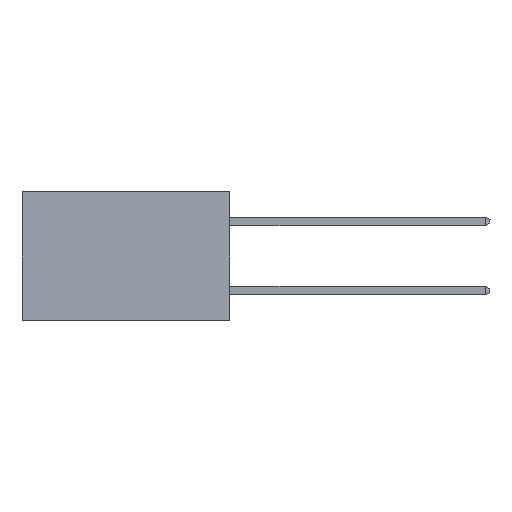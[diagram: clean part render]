
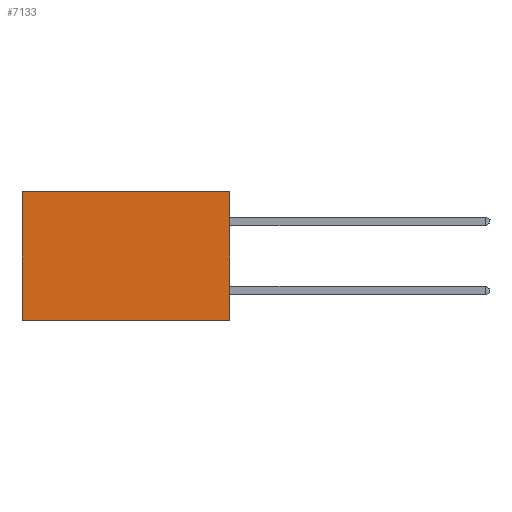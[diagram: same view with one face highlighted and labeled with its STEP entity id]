
A CAD part, left-side view. The second image highlights one B-rep face of the part: STEP entity #7133.
In plain terms, the highlighted planar face has unit normal (-1, 0, 0).
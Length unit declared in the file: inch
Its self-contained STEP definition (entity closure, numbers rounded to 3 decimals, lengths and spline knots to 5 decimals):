
#463 = ORIENTED_EDGE ( 'NONE', *, *, #21681, .F. ) ;
#1306 = FACE_OUTER_BOUND ( 'NONE', #14244, .T. ) ;
#1597 = VERTEX_POINT ( 'NONE', #17322 ) ;
#1683 = VECTOR ( 'NONE', #14192, 39.37008 ) ;
#1916 = PLANE ( 'NONE',  #7935 ) ;
#2069 = VERTEX_POINT ( 'NONE', #25078 ) ;
#2081 = LINE ( 'NONE', #17853, #12678 ) ;
#2197 = DIRECTION ( 'NONE',  ( 0., 0., -1. ) ) ;
#2674 = CARTESIAN_POINT ( 'NONE',  ( 0.2615, 0., -0.37 ) ) ;
#3080 = VECTOR ( 'NONE', #15954, 39.37008 ) ;
#6825 = VERTEX_POINT ( 'NONE', #20191 ) ;
#7133 = ADVANCED_FACE ( 'NONE', ( #1306 ), #1916, .F. ) ;
#7889 = ORIENTED_EDGE ( 'NONE', *, *, #12281, .T. ) ;
#7935 = AXIS2_PLACEMENT_3D ( 'NONE', #12000, #11866, #9193 ) ;
#8075 = CARTESIAN_POINT ( 'NONE',  ( 0.2615, 0., 0. ) ) ;
#9193 = DIRECTION ( 'NONE',  ( 0., 0., -1. ) ) ;
#11866 = DIRECTION ( 'NONE',  ( 1., 0., 0. ) ) ;
#12000 = CARTESIAN_POINT ( 'NONE',  ( 0.2615, 0., -0.37 ) ) ;
#12193 = LINE ( 'NONE', #8075, #3080 ) ;
#12235 = DIRECTION ( 'NONE',  ( 0., 0., -1. ) ) ;
#12281 = EDGE_CURVE ( 'NONE', #18769, #2069, #16241, .T. ) ;
#12386 = LINE ( 'NONE', #2674, #1683 ) ;
#12678 = VECTOR ( 'NONE', #2197, 39.37008 ) ;
#13939 = ORIENTED_EDGE ( 'NONE', *, *, #14836, .F. ) ;
#14192 = DIRECTION ( 'NONE',  ( 0., 1., 0. ) ) ;
#14244 = EDGE_LOOP ( 'NONE', ( #7889, #463, #13939, #14315 ) ) ;
#14315 = ORIENTED_EDGE ( 'NONE', *, *, #23627, .T. ) ;
#14667 = VECTOR ( 'NONE', #12235, 39.37008 ) ;
#14836 = EDGE_CURVE ( 'NONE', #1597, #6825, #2081, .T. ) ;
#15718 = CARTESIAN_POINT ( 'NONE',  ( 0.2615, 0.6, 0. ) ) ;
#15954 = DIRECTION ( 'NONE',  ( 0., 1., 0. ) ) ;
#16241 = LINE ( 'NONE', #16370, #14667 ) ;
#16370 = CARTESIAN_POINT ( 'NONE',  ( 0.2615, 0.6, -0.37 ) ) ;
#17322 = CARTESIAN_POINT ( 'NONE',  ( 0.2615, 0., 0. ) ) ;
#17853 = CARTESIAN_POINT ( 'NONE',  ( 0.2615, 0., -0.37 ) ) ;
#18769 = VERTEX_POINT ( 'NONE', #15718 ) ;
#20191 = CARTESIAN_POINT ( 'NONE',  ( 0.2615, 0., -0.37 ) ) ;
#21681 = EDGE_CURVE ( 'NONE', #6825, #2069, #12386, .T. ) ;
#23627 = EDGE_CURVE ( 'NONE', #1597, #18769, #12193, .T. ) ;
#25078 = CARTESIAN_POINT ( 'NONE',  ( 0.2615, 0.6, -0.37 ) ) ;
